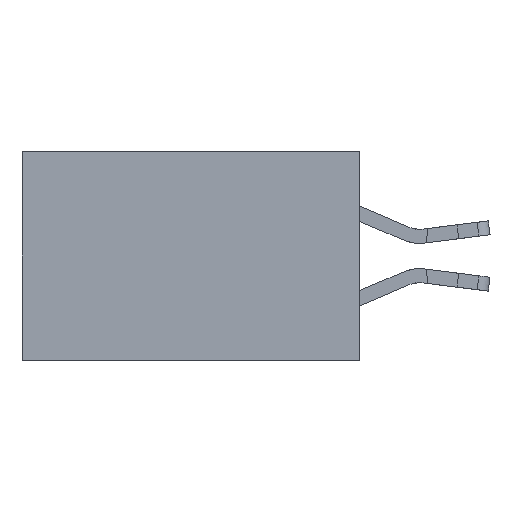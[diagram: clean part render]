
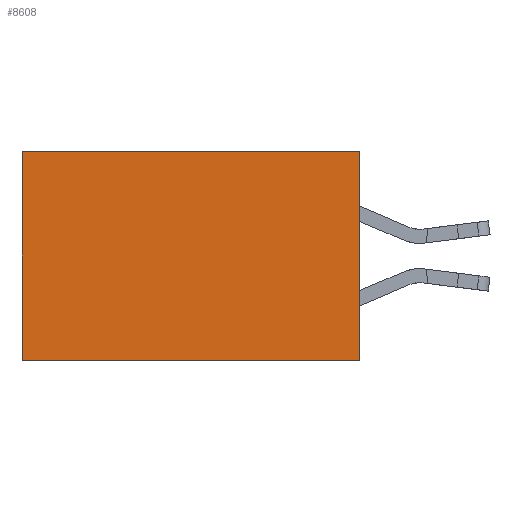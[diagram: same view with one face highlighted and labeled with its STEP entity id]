
A CAD part, left-side view. The second image highlights one B-rep face of the part: STEP entity #8608.
In plain terms, the highlighted planar face has unit normal (-1, 0, 0).
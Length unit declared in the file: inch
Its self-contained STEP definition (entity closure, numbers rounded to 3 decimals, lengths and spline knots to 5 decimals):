
#465 = DIRECTION ( 'NONE',  ( 0., 0., -1. ) ) ;
#1558 = ORIENTED_EDGE ( 'NONE', *, *, #21461, .T. ) ;
#2067 = CARTESIAN_POINT ( 'NONE',  ( 0.2875, 0., -0.37 ) ) ;
#4733 = PLANE ( 'NONE',  #14408 ) ;
#6048 = DIRECTION ( 'NONE',  ( 0., 1., 0. ) ) ;
#7049 = VECTOR ( 'NONE', #16270, 39.37008 ) ;
#7632 = DIRECTION ( 'NONE',  ( 0., 1., 0. ) ) ;
#8116 = ORIENTED_EDGE ( 'NONE', *, *, #13627, .T. ) ;
#8608 = ADVANCED_FACE ( 'NONE', ( #10307 ), #4733, .F. ) ;
#10214 = VERTEX_POINT ( 'NONE', #26401 ) ;
#10266 = DIRECTION ( 'NONE',  ( 0., 0., -1. ) ) ;
#10307 = FACE_OUTER_BOUND ( 'NONE', #22561, .T. ) ;
#10609 = CARTESIAN_POINT ( 'NONE',  ( 0.2875, 0.6, -0.37 ) ) ;
#10829 = ORIENTED_EDGE ( 'NONE', *, *, #25152, .F. ) ;
#12379 = CARTESIAN_POINT ( 'NONE',  ( 0.2875, 0., 0. ) ) ;
#13448 = LINE ( 'NONE', #12379, #23659 ) ;
#13627 = EDGE_CURVE ( 'NONE', #10214, #20106, #15618, .T. ) ;
#14408 = AXIS2_PLACEMENT_3D ( 'NONE', #17637, #21872, #465 ) ;
#14729 = VERTEX_POINT ( 'NONE', #17943 ) ;
#15618 = LINE ( 'NONE', #16010, #7049 ) ;
#16010 = CARTESIAN_POINT ( 'NONE',  ( 0.2875, 0.6, 0. ) ) ;
#16270 = DIRECTION ( 'NONE',  ( 0., 0., -1. ) ) ;
#17204 = CARTESIAN_POINT ( 'NONE',  ( 0.2875, 0., 0. ) ) ;
#17637 = CARTESIAN_POINT ( 'NONE',  ( 0.2875, 0., 0. ) ) ;
#17943 = CARTESIAN_POINT ( 'NONE',  ( 0.2875, 0., -0.37 ) ) ;
#18645 = VECTOR ( 'NONE', #6048, 39.37008 ) ;
#18689 = ORIENTED_EDGE ( 'NONE', *, *, #26330, .F. ) ;
#20106 = VERTEX_POINT ( 'NONE', #10609 ) ;
#21127 = VECTOR ( 'NONE', #7632, 39.37008 ) ;
#21156 = VERTEX_POINT ( 'NONE', #17204 ) ;
#21461 = EDGE_CURVE ( 'NONE', #21156, #10214, #25417, .T. ) ;
#21872 = DIRECTION ( 'NONE',  ( 1., 0., 0. ) ) ;
#22561 = EDGE_LOOP ( 'NONE', ( #8116, #18689, #10829, #1558 ) ) ;
#23228 = LINE ( 'NONE', #2067, #18645 ) ;
#23659 = VECTOR ( 'NONE', #10266, 39.37008 ) ;
#24207 = CARTESIAN_POINT ( 'NONE',  ( 0.2875, 0., 0. ) ) ;
#25152 = EDGE_CURVE ( 'NONE', #21156, #14729, #13448, .T. ) ;
#25417 = LINE ( 'NONE', #24207, #21127 ) ;
#26330 = EDGE_CURVE ( 'NONE', #14729, #20106, #23228, .T. ) ;
#26401 = CARTESIAN_POINT ( 'NONE',  ( 0.2875, 0.6, 0. ) ) ;
